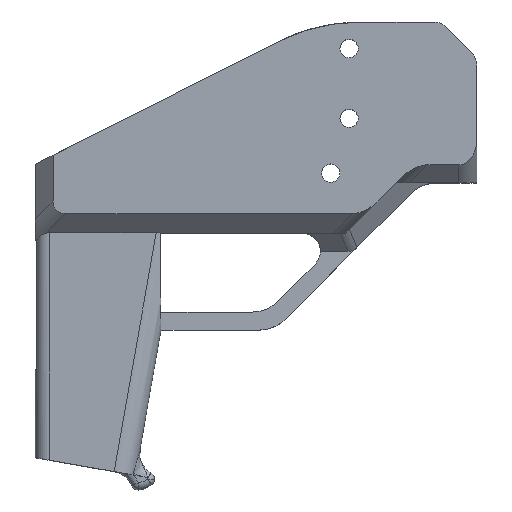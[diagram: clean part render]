
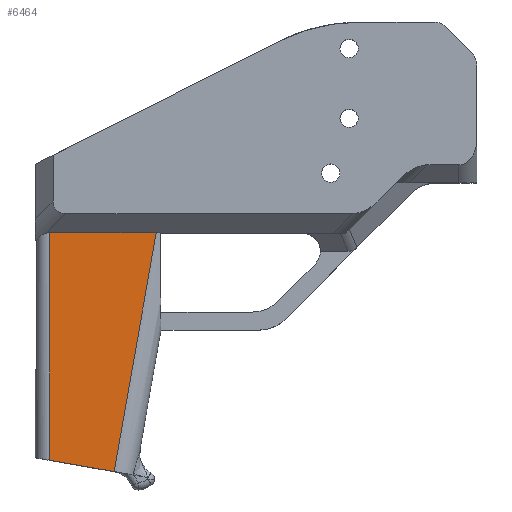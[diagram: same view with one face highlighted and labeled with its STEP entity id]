
A CAD part, top view. The second image highlights one B-rep face of the part: STEP entity #6464.
In plain terms, the highlighted planar face has unit normal (0, 0, 1).
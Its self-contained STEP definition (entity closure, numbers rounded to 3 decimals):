
#20 = VECTOR ( 'NONE', #3924, 1000. ) ;
#128 = EDGE_LOOP ( 'NONE', ( #6738, #3061, #1389, #6197 ) ) ;
#680 = VECTOR ( 'NONE', #1349, 1000. ) ;
#1009 = CARTESIAN_POINT ( 'NONE',  ( -122.937, -70., 35.32 ) ) ;
#1038 = PLANE ( 'NONE',  #2693 ) ;
#1093 = DIRECTION ( 'NONE',  ( 0.174, 0.985, 0. ) ) ;
#1318 = CARTESIAN_POINT ( 'NONE',  ( -122.937, 0.18, 35.32 ) ) ;
#1349 = DIRECTION ( 'NONE',  ( 0.985, -0.174, 0. ) ) ;
#1389 = ORIENTED_EDGE ( 'NONE', *, *, #3230, .T. ) ;
#1649 = DIRECTION ( 'NONE',  ( -1., 0., 0. ) ) ;
#1964 = CARTESIAN_POINT ( 'NONE',  ( -118.937, -63.123, 35.32 ) ) ;
#2303 = LINE ( 'NONE', #3108, #680 ) ;
#2318 = CARTESIAN_POINT ( 'NONE',  ( -93.846, -25.958, 35.32 ) ) ;
#2495 = VECTOR ( 'NONE', #5571, 1000. ) ;
#2682 = VERTEX_POINT ( 'NONE', #7690 ) ;
#2693 = AXIS2_PLACEMENT_3D ( 'NONE', #1009, #5292, #1649 ) ;
#2749 = EDGE_CURVE ( 'NONE', #4151, #5213, #3719, .T. ) ;
#3061 = ORIENTED_EDGE ( 'NONE', *, *, #7138, .T. ) ;
#3108 = CARTESIAN_POINT ( 'NONE',  ( -79.937, -70., 35.32 ) ) ;
#3198 = EDGE_CURVE ( 'NONE', #5213, #2682, #5910, .T. ) ;
#3228 = VERTEX_POINT ( 'NONE', #1964 ) ;
#3230 = EDGE_CURVE ( 'NONE', #3228, #4151, #2303, .T. ) ;
#3719 = LINE ( 'NONE', #2318, #6768 ) ;
#3762 = CARTESIAN_POINT ( 'NONE',  ( -89.237, 0.18, 35.32 ) ) ;
#3924 = DIRECTION ( 'NONE',  ( 0., -1., 0. ) ) ;
#4151 = VERTEX_POINT ( 'NONE', #4196 ) ;
#4196 = CARTESIAN_POINT ( 'NONE',  ( -100.958, -66.293, 35.32 ) ) ;
#5159 = CARTESIAN_POINT ( 'NONE',  ( -118.937, -62.418, 35.32 ) ) ;
#5213 = VERTEX_POINT ( 'NONE', #3762 ) ;
#5292 = DIRECTION ( 'NONE',  ( 0., 0., -1. ) ) ;
#5571 = DIRECTION ( 'NONE',  ( -1., 0., 0. ) ) ;
#5910 = LINE ( 'NONE', #1318, #2495 ) ;
#6197 = ORIENTED_EDGE ( 'NONE', *, *, #2749, .T. ) ;
#6318 = LINE ( 'NONE', #5159, #20 ) ;
#6464 = ADVANCED_FACE ( 'NONE', ( #6891 ), #1038, .F. ) ;
#6738 = ORIENTED_EDGE ( 'NONE', *, *, #3198, .T. ) ;
#6768 = VECTOR ( 'NONE', #1093, 1000. ) ;
#6891 = FACE_OUTER_BOUND ( 'NONE', #128, .T. ) ;
#7138 = EDGE_CURVE ( 'NONE', #2682, #3228, #6318, .T. ) ;
#7690 = CARTESIAN_POINT ( 'NONE',  ( -118.937, 0.18, 35.32 ) ) ;
